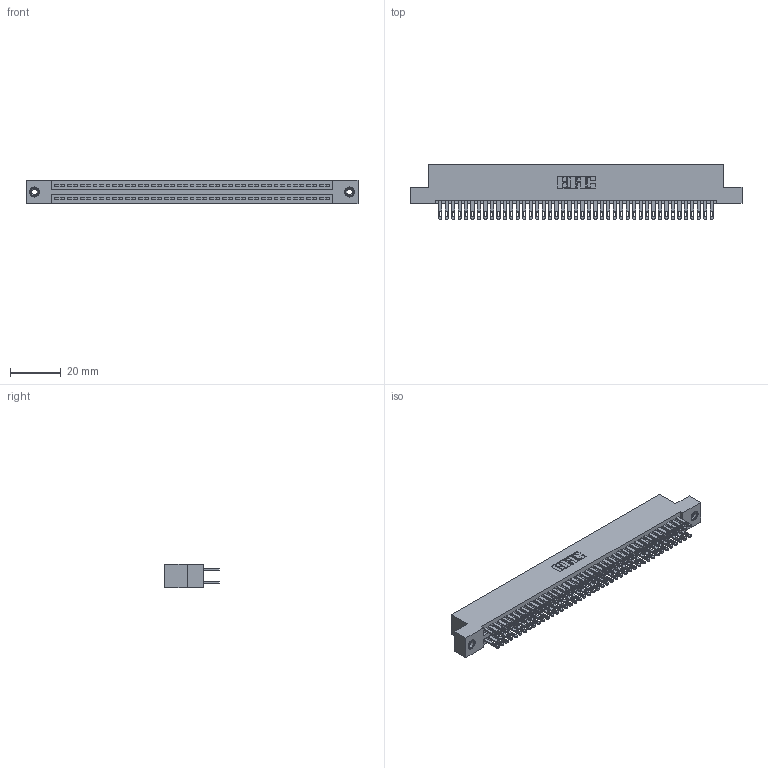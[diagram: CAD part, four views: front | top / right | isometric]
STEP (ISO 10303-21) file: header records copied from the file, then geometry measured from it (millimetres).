
FILE_DESCRIPTION (( 'STEP AP203' ), '1' );
FILE_NAME ('345-086-500-208.STEP', '2019-11-01T06:14:04', ( '' ), ( '' ), 'SwSTEP 2.0', 'SolidWorks 2016', '' );
FILE_SCHEMA (( 'CONFIG_CONTROL_DESIGN' ));
Length unit declared in the file: inch
Products named in the file (4): 345-250-001_345-250-003-102; 345-086-500-208; 345 Part_Flush Mounting Lugs - 0.156 Dia-TI; 345-292-001_345-293-100
Assembly tree (89 placements, depth 2):
  345-086-500-208
    345 Part_Flush Mounting Lugs - 0.156 Dia-TI
    345-292-001_345-293-100  x86
    345-250-001_345-250-003-102  x2
Bounding box: 130.43 x 21.51 x 9.4 mm (x, y, z)
Volume: 12935.6 mm3; surface area: 20030.9 mm2
Topology: 89 solids, 89 shells, 4142 faces, 12603 edges, 8394 vertices
Faces by surface type: plane 2434, cylinder 1692, cone 12, torus 4
Entity records: 34720 total; most frequent: CARTESIAN_POINT 5799, ORIENTED_EDGE 5726, DIRECTION 5141, EDGE_CURVE 2863, VECTOR 2535, LINE 2535, VERTEX_POINT 1904, AXIS2_PLACEMENT_3D 1303
